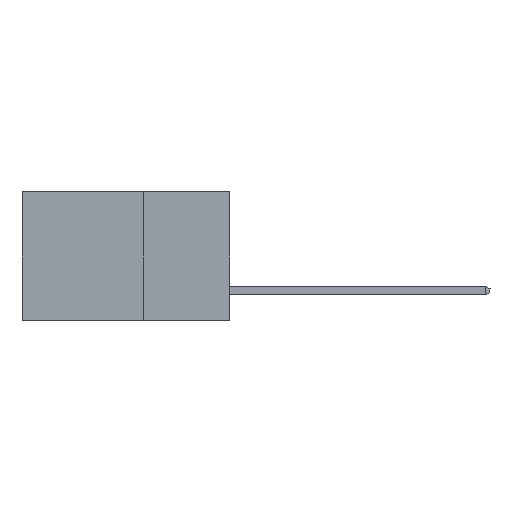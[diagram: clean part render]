
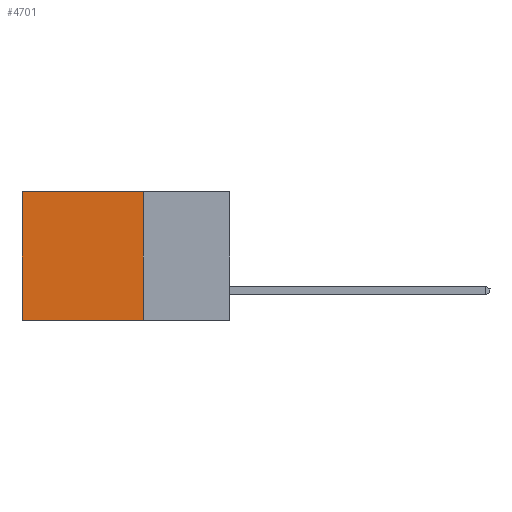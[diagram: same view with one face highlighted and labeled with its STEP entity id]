
A CAD part, left-side view. The second image highlights one B-rep face of the part: STEP entity #4701.
In plain terms, the highlighted planar face has unit normal (-1, 0, 0).
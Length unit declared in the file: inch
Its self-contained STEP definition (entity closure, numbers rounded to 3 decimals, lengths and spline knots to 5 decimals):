
#129 = LINE ( 'NONE', #18167, #4687 ) ;
#531 = PLANE ( 'NONE',  #20782 ) ;
#587 = DIRECTION ( 'NONE',  ( 0., 0., -1. ) ) ;
#2301 = CARTESIAN_POINT ( 'NONE',  ( 0.2615, 0.25, -0.37 ) ) ;
#2646 = FACE_OUTER_BOUND ( 'NONE', #23899, .T. ) ;
#2739 = CARTESIAN_POINT ( 'NONE',  ( 0.2615, 0.25, 0. ) ) ;
#3506 = CARTESIAN_POINT ( 'NONE',  ( 0.2615, 0.6, 0. ) ) ;
#4650 = DIRECTION ( 'NONE',  ( 0., 0., -1. ) ) ;
#4687 = VECTOR ( 'NONE', #8226, 39.37008 ) ;
#4701 = ADVANCED_FACE ( 'NONE', ( #2646 ), #531, .F. ) ;
#6014 = ORIENTED_EDGE ( 'NONE', *, *, #21789, .F. ) ;
#7056 = VERTEX_POINT ( 'NONE', #9089 ) ;
#7794 = CARTESIAN_POINT ( 'NONE',  ( 0.2615, 0.25, -0.37 ) ) ;
#8226 = DIRECTION ( 'NONE',  ( 0., 0., -1. ) ) ;
#8453 = ORIENTED_EDGE ( 'NONE', *, *, #8669, .T. ) ;
#8669 = EDGE_CURVE ( 'NONE', #24412, #13430, #10974, .T. ) ;
#8713 = DIRECTION ( 'NONE',  ( 0., 1., 0. ) ) ;
#9089 = CARTESIAN_POINT ( 'NONE',  ( 0.2615, 0.6, -0.37 ) ) ;
#9905 = DIRECTION ( 'NONE',  ( 0., 1., 0. ) ) ;
#10734 = DIRECTION ( 'NONE',  ( 1., 0., 0. ) ) ;
#10974 = LINE ( 'NONE', #2739, #24318 ) ;
#12012 = ORIENTED_EDGE ( 'NONE', *, *, #18613, .T. ) ;
#12379 = LINE ( 'NONE', #2301, #25458 ) ;
#13430 = VERTEX_POINT ( 'NONE', #3506 ) ;
#14313 = CARTESIAN_POINT ( 'NONE',  ( 0.2615, 0.25, -0.37 ) ) ;
#14704 = VERTEX_POINT ( 'NONE', #21407 ) ;
#18167 = CARTESIAN_POINT ( 'NONE',  ( 0.2615, 0.6, -0.37 ) ) ;
#18613 = EDGE_CURVE ( 'NONE', #13430, #7056, #129, .T. ) ;
#19576 = EDGE_CURVE ( 'NONE', #24412, #14704, #12379, .T. ) ;
#20782 = AXIS2_PLACEMENT_3D ( 'NONE', #14313, #10734, #4650 ) ;
#20786 = ORIENTED_EDGE ( 'NONE', *, *, #19576, .F. ) ;
#21180 = CARTESIAN_POINT ( 'NONE',  ( 0.2615, 0.25, 0. ) ) ;
#21407 = CARTESIAN_POINT ( 'NONE',  ( 0.2615, 0.25, -0.37 ) ) ;
#21705 = LINE ( 'NONE', #7794, #23814 ) ;
#21789 = EDGE_CURVE ( 'NONE', #14704, #7056, #21705, .T. ) ;
#23814 = VECTOR ( 'NONE', #9905, 39.37008 ) ;
#23899 = EDGE_LOOP ( 'NONE', ( #12012, #6014, #20786, #8453 ) ) ;
#24318 = VECTOR ( 'NONE', #8713, 39.37008 ) ;
#24412 = VERTEX_POINT ( 'NONE', #21180 ) ;
#25458 = VECTOR ( 'NONE', #587, 39.37008 ) ;
